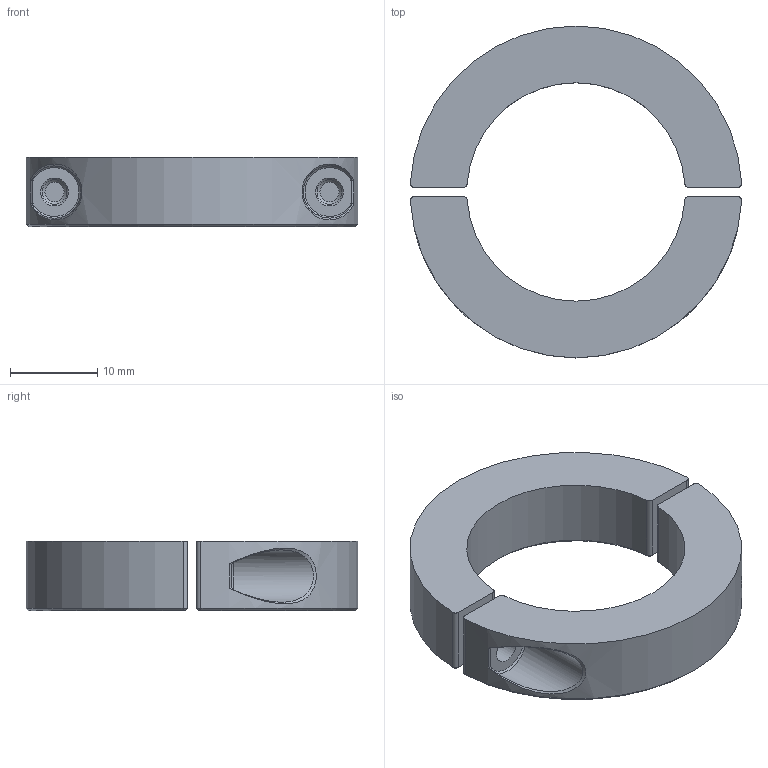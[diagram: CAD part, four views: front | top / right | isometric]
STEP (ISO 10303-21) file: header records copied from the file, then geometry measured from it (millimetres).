
FILE_DESCRIPTION(/* description */ (''),/* implementation_level */ '2;1');
FILE_NAME(/* name */ 'suppressor_blast_deflector.step',/* time_stamp */ '2024-04-08T19:46:50+12:00',/* author */ (''),/* organization */ (''),/* preprocessor_version */ 'ST-DEVELOPER v20',/* originating_system */ 'Autodesk Translation Framework v12.20.1.177',/* authorisation */ '');
FILE_SCHEMA (('AUTOMOTIVE_DESIGN { 1 0 10303 214 3 1 1 }'));
Length unit declared in the file: millimetre
Products named in the file (1): suppressor_blast_deflector
Bounding box: 37.94 x 38 x 8 mm (x, y, z)
Volume: 4563.5 mm3; surface area: 3251.2 mm2
Topology: 2 solids, 2 shells, 62 faces, 128 edges, 74 vertices
Faces by surface type: plane 22, cone 20, cylinder 18, bspline 2
Full cylindrical faces by diameter (mm): 2.8 x2, 3.2 x2
Entity records: 2368 total; most frequent: CARTESIAN_POINT 1024, DIRECTION 292, ORIENTED_EDGE 256, EDGE_CURVE 128, AXIS2_PLACEMENT_3D 115, VERTEX_POINT 74, EDGE_LOOP 70, FACE_OUTER_BOUND 62
